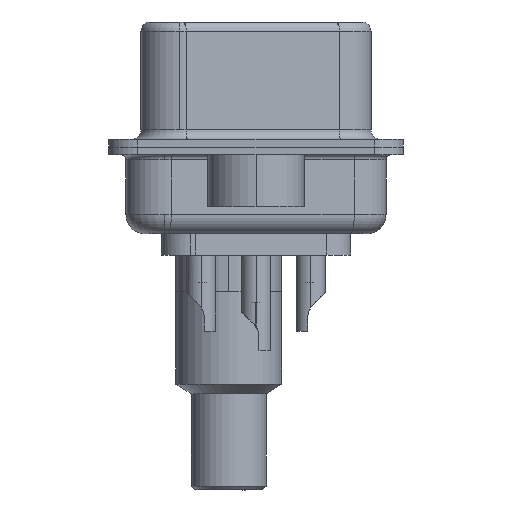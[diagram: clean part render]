
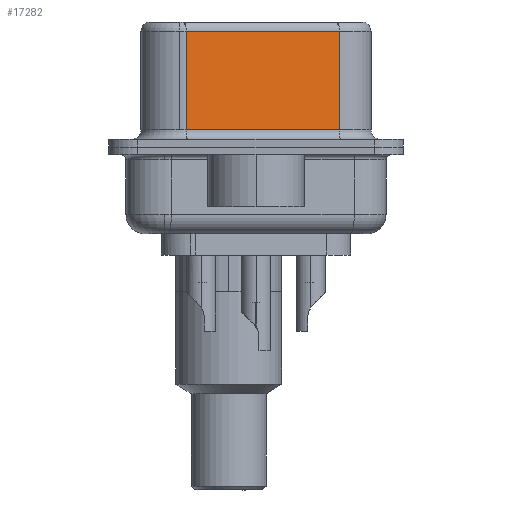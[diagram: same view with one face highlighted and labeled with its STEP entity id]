
A CAD part, left-side view. The second image highlights one B-rep face of the part: STEP entity #17282.
In plain terms, the highlighted planar face has unit normal (-0.985, -0.174, 0).
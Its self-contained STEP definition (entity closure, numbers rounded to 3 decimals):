
#365 = VECTOR ( 'NONE', #28938, 1000. ) ;
#670 = ORIENTED_EDGE ( 'NONE', *, *, #16739, .F. ) ;
#1662 = DIRECTION ( 'NONE',  ( 0.174, -0.985, 0. ) ) ;
#2347 = LINE ( 'NONE', #6190, #365 ) ;
#2576 = CARTESIAN_POINT ( 'NONE',  ( 5.132, -4.322, 6.52 ) ) ;
#3548 = EDGE_CURVE ( 'NONE', #19466, #17139, #2347, .T. ) ;
#3852 = EDGE_LOOP ( 'NONE', ( #670, #22079, #7462, #9971 ) ) ;
#4934 = DIRECTION ( 'NONE',  ( 0.985, 0.174, 0. ) ) ;
#6190 = CARTESIAN_POINT ( 'NONE',  ( 5.132, -4.322, 6.02 ) ) ;
#7103 = EDGE_CURVE ( 'NONE', #15692, #12690, #8171, .T. ) ;
#7462 = ORIENTED_EDGE ( 'NONE', *, *, #9831, .T. ) ;
#8171 = LINE ( 'NONE', #14330, #18549 ) ;
#8745 = CARTESIAN_POINT ( 'NONE',  ( 3.73, 3.628, 0.9 ) ) ;
#9205 = LINE ( 'NONE', #11830, #26849 ) ;
#9831 = EDGE_CURVE ( 'NONE', #17139, #15692, #9205, .T. ) ;
#9971 = ORIENTED_EDGE ( 'NONE', *, *, #7103, .T. ) ;
#10299 = VECTOR ( 'NONE', #24920, 1000. ) ;
#11830 = CARTESIAN_POINT ( 'NONE',  ( 3.73, 3.628, 6.52 ) ) ;
#11861 = CARTESIAN_POINT ( 'NONE',  ( 5.132, -4.322, 6.52 ) ) ;
#12690 = VERTEX_POINT ( 'NONE', #27361 ) ;
#14330 = CARTESIAN_POINT ( 'NONE',  ( 5.132, -4.322, 0.9 ) ) ;
#15692 = VERTEX_POINT ( 'NONE', #8745 ) ;
#16739 = EDGE_CURVE ( 'NONE', #19466, #12690, #29140, .T. ) ;
#17139 = VERTEX_POINT ( 'NONE', #25304 ) ;
#17282 = ADVANCED_FACE ( 'NONE', ( #21113 ), #17942, .F. ) ;
#17942 = PLANE ( 'NONE',  #32112 ) ;
#18549 = VECTOR ( 'NONE', #1662, 1000. ) ;
#19466 = VERTEX_POINT ( 'NONE', #19801 ) ;
#19801 = CARTESIAN_POINT ( 'NONE',  ( 5.132, -4.322, 6.02 ) ) ;
#20727 = DIRECTION ( 'NONE',  ( -0.174, 0.985, 0. ) ) ;
#21113 = FACE_OUTER_BOUND ( 'NONE', #3852, .T. ) ;
#22079 = ORIENTED_EDGE ( 'NONE', *, *, #3548, .T. ) ;
#24920 = DIRECTION ( 'NONE',  ( 0., 0., -1. ) ) ;
#25304 = CARTESIAN_POINT ( 'NONE',  ( 3.73, 3.628, 6.02 ) ) ;
#26849 = VECTOR ( 'NONE', #29773, 1000. ) ;
#27361 = CARTESIAN_POINT ( 'NONE',  ( 5.132, -4.322, 0.9 ) ) ;
#28938 = DIRECTION ( 'NONE',  ( -0.174, 0.985, 0. ) ) ;
#29140 = LINE ( 'NONE', #11861, #10299 ) ;
#29773 = DIRECTION ( 'NONE',  ( 0., 0., -1. ) ) ;
#32112 = AXIS2_PLACEMENT_3D ( 'NONE', #2576, #4934, #20727 ) ;
